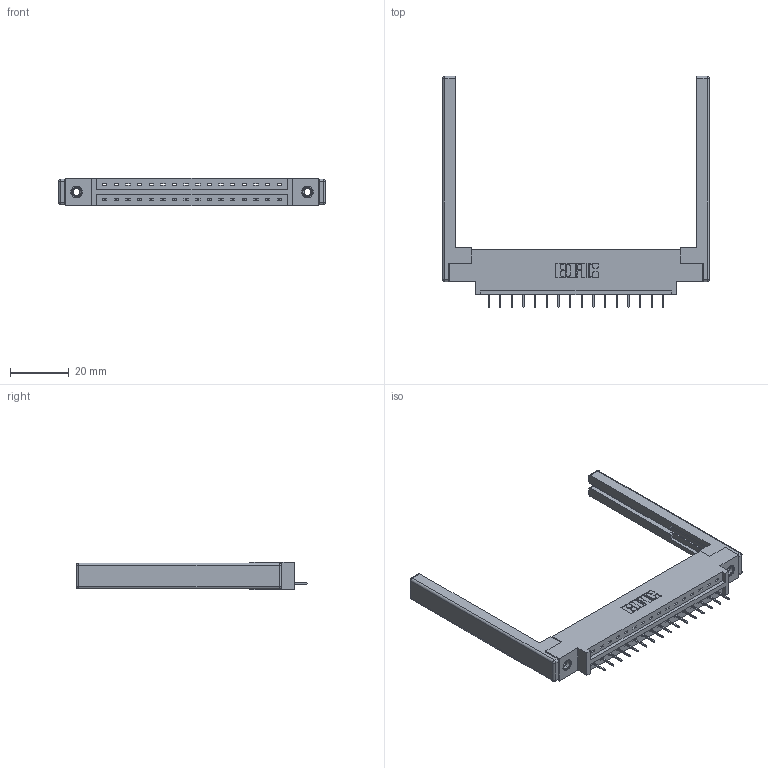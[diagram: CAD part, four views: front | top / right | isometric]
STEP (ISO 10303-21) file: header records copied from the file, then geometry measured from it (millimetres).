
FILE_DESCRIPTION (( 'STEP AP203' ), '1' );
FILE_NAME ('337-016-524-668.STEP', '2019-09-28T17:39:48', ( '' ), ( '' ), 'SwSTEP 2.0', 'SolidWorks 2016', '' );
FILE_SCHEMA (( 'CONFIG_CONTROL_DESIGN' ));
Length unit declared in the file: inch
Products named in the file (5): 337 Part_0.170 Offset - 0.156 Dia-TI; 337-016-524-668; 307-220-068; 345-250-001_345-250-001-102; 345-292-001_345-293-124
Assembly tree (21 placements, depth 2):
  337-016-524-668
    337 Part_0.170 Offset - 0.156 Dia-TI
    345-292-001_345-293-124  x16
    345-250-001_345-250-001-102  x2
    307-220-068  x2
Bounding box: 90.83 x 78.75 x 9.4 mm (x, y, z)
Volume: 13325.4 mm3; surface area: 13054.7 mm2
Topology: 21 solids, 21 shells, 1328 faces, 3785 edges, 2438 vertices
Faces by surface type: plane 994, cylinder 310, cone 12, sphere 8, torus 4
Entity records: 18222 total; most frequent: CARTESIAN_POINT 3127, ORIENTED_EDGE 3068, DIRECTION 2760, EDGE_CURVE 1534, LINE 1360, VECTOR 1360, VERTEX_POINT 1010, AXIS2_PLACEMENT_3D 700
